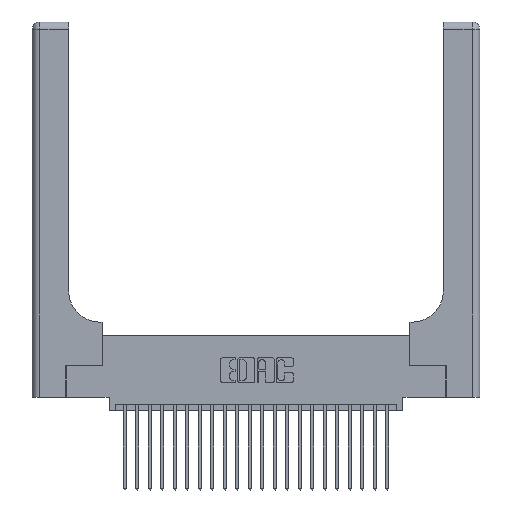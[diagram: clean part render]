
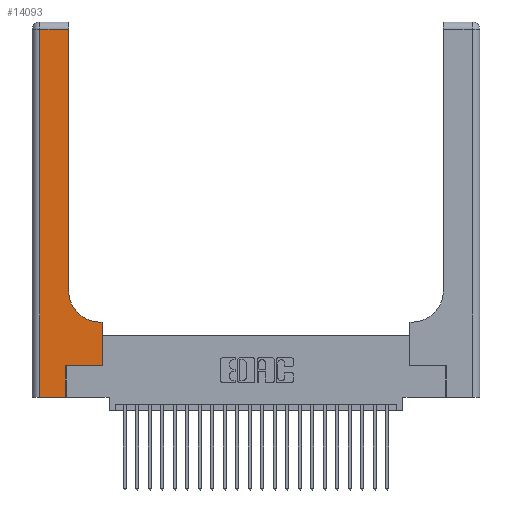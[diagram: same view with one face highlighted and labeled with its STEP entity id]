
A CAD part, top view. The second image highlights one B-rep face of the part: STEP entity #14093.
In plain terms, the highlighted planar face has unit normal (0, 0, 1).
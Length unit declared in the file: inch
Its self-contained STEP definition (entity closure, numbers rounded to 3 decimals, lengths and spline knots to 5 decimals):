
#251 = VERTEX_POINT ( 'NONE', #5222 ) ;
#471 = DIRECTION ( 'NONE',  ( -1., 0., 0. ) ) ;
#514 = VECTOR ( 'NONE', #19361, 39.37008 ) ;
#620 = CARTESIAN_POINT ( 'NONE',  ( 0.5585, 0.25, 0.37 ) ) ;
#757 = EDGE_CURVE ( 'NONE', #251, #5807, #7159, .T. ) ;
#856 = DIRECTION ( 'NONE',  ( -1., 0., 0. ) ) ;
#1509 = CARTESIAN_POINT ( 'NONE',  ( 0., 2.94, 0.37 ) ) ;
#1781 = ORIENTED_EDGE ( 'NONE', *, *, #4631, .T. ) ;
#1865 = VECTOR ( 'NONE', #856, 39.37008 ) ;
#1875 = LINE ( 'NONE', #7095, #6566 ) ;
#2184 = LINE ( 'NONE', #17970, #12118 ) ;
#2412 = CARTESIAN_POINT ( 'NONE',  ( 0., 3., 0.37 ) ) ;
#2508 = DIRECTION ( 'NONE',  ( -1., 0., 0. ) ) ;
#3778 = CARTESIAN_POINT ( 'NONE',  ( 0.2915, 3., 0.37 ) ) ;
#3969 = ORIENTED_EDGE ( 'NONE', *, *, #21120, .T. ) ;
#4631 = EDGE_CURVE ( 'NONE', #9179, #19649, #11875, .T. ) ;
#4867 = VERTEX_POINT ( 'NONE', #7273 ) ;
#4944 = CARTESIAN_POINT ( 'NONE',  ( 0.2915, 0.85, 0.37 ) ) ;
#4948 = VECTOR ( 'NONE', #5742, 39.37008 ) ;
#5222 = CARTESIAN_POINT ( 'NONE',  ( 0.2915, 2.94, 0.37 ) ) ;
#5742 = DIRECTION ( 'NONE',  ( 0., -1., 0. ) ) ;
#5807 = VERTEX_POINT ( 'NONE', #16097 ) ;
#5841 = EDGE_CURVE ( 'NONE', #19649, #4867, #17219, .T. ) ;
#5853 = ORIENTED_EDGE ( 'NONE', *, *, #18726, .T. ) ;
#6018 = EDGE_LOOP ( 'NONE', ( #3969, #9842, #25234, #5853, #21326, #16824, #1781, #12323, #12940 ) ) ;
#6119 = CARTESIAN_POINT ( 'NONE',  ( 0.269, 0., 0.37 ) ) ;
#6559 = CARTESIAN_POINT ( 'NONE',  ( 0.06, 0., 0.37 ) ) ;
#6562 = CARTESIAN_POINT ( 'NONE',  ( 0.5415, 0.85, 0.37 ) ) ;
#6566 = VECTOR ( 'NONE', #22580, 39.37008 ) ;
#6975 = CARTESIAN_POINT ( 'NONE',  ( 0.269, 0.25, 0.37 ) ) ;
#7095 = CARTESIAN_POINT ( 'NONE',  ( 0.269, 0.25, 0.37 ) ) ;
#7159 = LINE ( 'NONE', #1509, #1865 ) ;
#7221 = VECTOR ( 'NONE', #8012, 39.37008 ) ;
#7252 = VECTOR ( 'NONE', #12537, 39.37008 ) ;
#7273 = CARTESIAN_POINT ( 'NONE',  ( 0.5415, 0.6, 0.37 ) ) ;
#7503 = VECTOR ( 'NONE', #2508, 39.37008 ) ;
#8012 = DIRECTION ( 'NONE',  ( 0., 1., 0. ) ) ;
#8523 = DIRECTION ( 'NONE',  ( 1., 0., 0. ) ) ;
#8723 = CARTESIAN_POINT ( 'NONE',  ( 0.269, 0., 0.37 ) ) ;
#9179 = VERTEX_POINT ( 'NONE', #17872 ) ;
#9842 = ORIENTED_EDGE ( 'NONE', *, *, #757, .T. ) ;
#10202 = LINE ( 'NONE', #19300, #4948 ) ;
#10223 = VERTEX_POINT ( 'NONE', #6975 ) ;
#11183 = CARTESIAN_POINT ( 'NONE',  ( 0.5585, 0.6, 0.37 ) ) ;
#11720 = FACE_OUTER_BOUND ( 'NONE', #6018, .T. ) ;
#11875 = LINE ( 'NONE', #620, #7252 ) ;
#12118 = VECTOR ( 'NONE', #19898, 39.37008 ) ;
#12323 = ORIENTED_EDGE ( 'NONE', *, *, #5841, .T. ) ;
#12385 = DIRECTION ( 'NONE',  ( 0., 0., -1. ) ) ;
#12537 = DIRECTION ( 'NONE',  ( 0., 1., 0. ) ) ;
#12940 = ORIENTED_EDGE ( 'NONE', *, *, #15864, .T. ) ;
#14093 = ADVANCED_FACE ( 'NONE', ( #11720 ), #19991, .F. ) ;
#14330 = CARTESIAN_POINT ( 'NONE',  ( 0.2915, 0.6, 0.37 ) ) ;
#14656 = VERTEX_POINT ( 'NONE', #4944 ) ;
#15864 = EDGE_CURVE ( 'NONE', #4867, #14656, #20349, .T. ) ;
#16097 = CARTESIAN_POINT ( 'NONE',  ( 0.06, 2.94, 0.37 ) ) ;
#16260 = LINE ( 'NONE', #3778, #514 ) ;
#16824 = ORIENTED_EDGE ( 'NONE', *, *, #18986, .T. ) ;
#16948 = LINE ( 'NONE', #6119, #7221 ) ;
#17219 = LINE ( 'NONE', #14330, #7503 ) ;
#17872 = CARTESIAN_POINT ( 'NONE',  ( 0.5585, 0.25, 0.37 ) ) ;
#17970 = CARTESIAN_POINT ( 'NONE',  ( 0., 0., 0.37 ) ) ;
#18082 = EDGE_CURVE ( 'NONE', #22968, #10223, #16948, .T. ) ;
#18726 = EDGE_CURVE ( 'NONE', #23979, #22968, #2184, .T. ) ;
#18986 = EDGE_CURVE ( 'NONE', #10223, #9179, #1875, .T. ) ;
#19300 = CARTESIAN_POINT ( 'NONE',  ( 0.06, 3., 0.37 ) ) ;
#19361 = DIRECTION ( 'NONE',  ( 0., 1., 0. ) ) ;
#19649 = VERTEX_POINT ( 'NONE', #11183 ) ;
#19898 = DIRECTION ( 'NONE',  ( 1., 0., 0. ) ) ;
#19991 = PLANE ( 'NONE',  #24394 ) ;
#20101 = DIRECTION ( 'NONE',  ( 0., 0., -1. ) ) ;
#20349 = CIRCLE ( 'NONE', #24567, 0.25 ) ;
#21120 = EDGE_CURVE ( 'NONE', #14656, #251, #16260, .T. ) ;
#21326 = ORIENTED_EDGE ( 'NONE', *, *, #18082, .T. ) ;
#22220 = EDGE_CURVE ( 'NONE', #5807, #23979, #10202, .T. ) ;
#22580 = DIRECTION ( 'NONE',  ( 1., 0., 0. ) ) ;
#22968 = VERTEX_POINT ( 'NONE', #8723 ) ;
#23979 = VERTEX_POINT ( 'NONE', #6559 ) ;
#24394 = AXIS2_PLACEMENT_3D ( 'NONE', #2412, #12385, #471 ) ;
#24567 = AXIS2_PLACEMENT_3D ( 'NONE', #6562, #20101, #8523 ) ;
#25234 = ORIENTED_EDGE ( 'NONE', *, *, #22220, .T. ) ;
